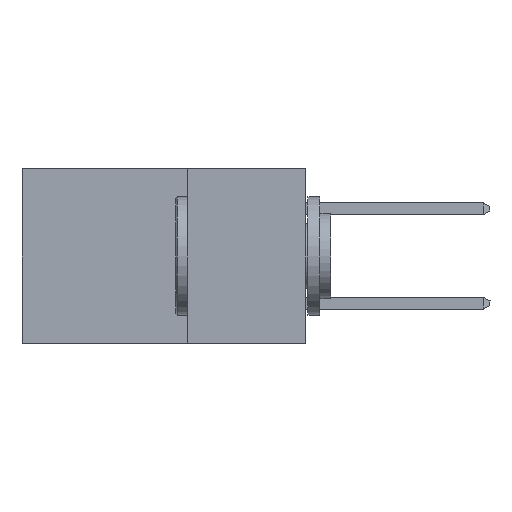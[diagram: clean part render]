
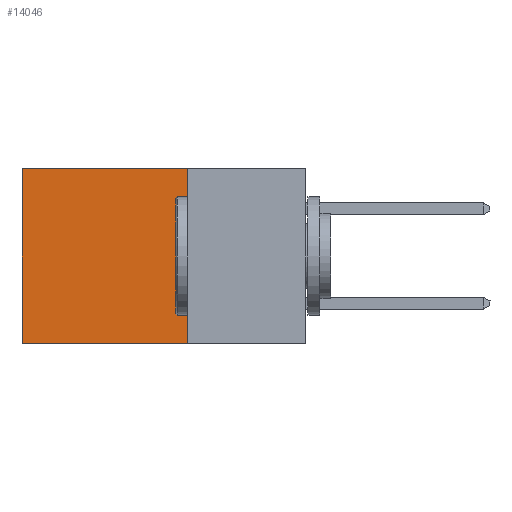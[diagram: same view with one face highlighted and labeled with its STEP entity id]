
A CAD part, left-side view. The second image highlights one B-rep face of the part: STEP entity #14046.
In plain terms, the highlighted planar face has unit normal (-1, 0, 0).
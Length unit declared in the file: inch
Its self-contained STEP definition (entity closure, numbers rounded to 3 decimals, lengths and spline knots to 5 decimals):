
#146 = EDGE_CURVE ( 'NONE', #15729, #5535, #15338, .T. ) ;
#212 = DIRECTION ( 'NONE',  ( 0., 0., -1. ) ) ;
#255 = DIRECTION ( 'NONE',  ( 1., 0., 0. ) ) ;
#489 = CARTESIAN_POINT ( 'NONE',  ( 0.2615, 0.25, -0.37 ) ) ;
#512 = PLANE ( 'NONE',  #11989 ) ;
#857 = VECTOR ( 'NONE', #1591, 39.37008 ) ;
#1082 = CARTESIAN_POINT ( 'NONE',  ( 0.2615, 0.25, -0.37 ) ) ;
#1582 = EDGE_CURVE ( 'NONE', #13547, #6474, #6896, .T. ) ;
#1591 = DIRECTION ( 'NONE',  ( 0., 1., 0. ) ) ;
#1611 = CARTESIAN_POINT ( 'NONE',  ( 0.2615, 0.25, 0. ) ) ;
#2148 = DIRECTION ( 'NONE',  ( 0., 0., -1. ) ) ;
#2226 = VECTOR ( 'NONE', #2148, 39.37008 ) ;
#3961 = ORIENTED_EDGE ( 'NONE', *, *, #8514, .T. ) ;
#5535 = VERTEX_POINT ( 'NONE', #9231 ) ;
#6474 = VERTEX_POINT ( 'NONE', #14989 ) ;
#6825 = ORIENTED_EDGE ( 'NONE', *, *, #1582, .T. ) ;
#6896 = LINE ( 'NONE', #7553, #13085 ) ;
#6974 = EDGE_CURVE ( 'NONE', #5535, #6474, #14634, .T. ) ;
#7143 = ORIENTED_EDGE ( 'NONE', *, *, #6974, .F. ) ;
#7526 = LINE ( 'NONE', #1611, #857 ) ;
#7553 = CARTESIAN_POINT ( 'NONE',  ( 0.2615, 0.6, -0.37 ) ) ;
#8514 = EDGE_CURVE ( 'NONE', #15729, #13547, #7526, .T. ) ;
#9231 = CARTESIAN_POINT ( 'NONE',  ( 0.2615, 0.25, -0.37 ) ) ;
#9744 = CARTESIAN_POINT ( 'NONE',  ( 0.2615, 0.25, 0. ) ) ;
#10417 = ORIENTED_EDGE ( 'NONE', *, *, #146, .F. ) ;
#10804 = CARTESIAN_POINT ( 'NONE',  ( 0.2615, 0.6, 0. ) ) ;
#11065 = VECTOR ( 'NONE', #11825, 39.37008 ) ;
#11825 = DIRECTION ( 'NONE',  ( 0., 1., 0. ) ) ;
#11981 = CARTESIAN_POINT ( 'NONE',  ( 0.2615, 0.25, -0.37 ) ) ;
#11989 = AXIS2_PLACEMENT_3D ( 'NONE', #489, #255, #212 ) ;
#12368 = EDGE_LOOP ( 'NONE', ( #6825, #7143, #10417, #3961 ) ) ;
#12532 = FACE_OUTER_BOUND ( 'NONE', #12368, .T. ) ;
#13085 = VECTOR ( 'NONE', #15413, 39.37008 ) ;
#13547 = VERTEX_POINT ( 'NONE', #10804 ) ;
#14046 = ADVANCED_FACE ( 'NONE', ( #12532 ), #512, .F. ) ;
#14634 = LINE ( 'NONE', #11981, #11065 ) ;
#14989 = CARTESIAN_POINT ( 'NONE',  ( 0.2615, 0.6, -0.37 ) ) ;
#15338 = LINE ( 'NONE', #1082, #2226 ) ;
#15413 = DIRECTION ( 'NONE',  ( 0., 0., -1. ) ) ;
#15729 = VERTEX_POINT ( 'NONE', #9744 ) ;
